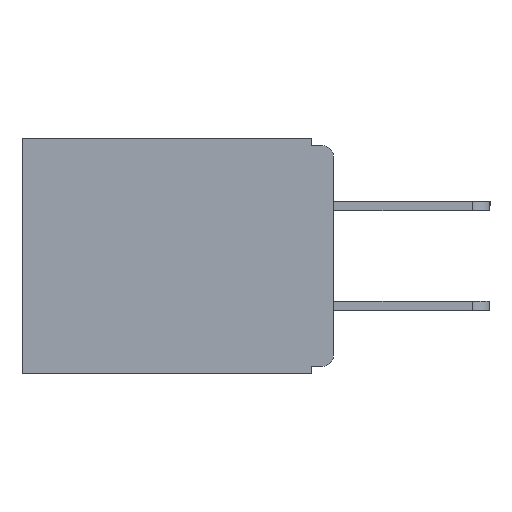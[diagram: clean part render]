
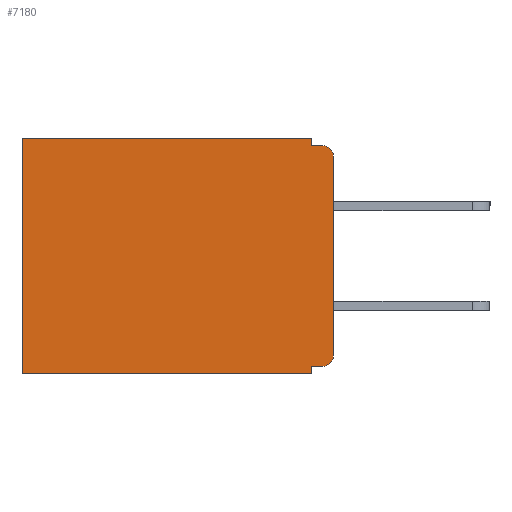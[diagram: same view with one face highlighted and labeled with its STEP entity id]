
A CAD part, left-side view. The second image highlights one B-rep face of the part: STEP entity #7180.
In plain terms, the highlighted planar face has unit normal (-1, 0, 0).
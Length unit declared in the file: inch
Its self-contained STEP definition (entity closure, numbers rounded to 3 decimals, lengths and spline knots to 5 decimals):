
#23 = ORIENTED_EDGE ( 'NONE', *, *, #28409, .T. ) ;
#309 = CARTESIAN_POINT ( 'NONE',  ( 0.3, 0.437, -0.33 ) ) ;
#776 = CARTESIAN_POINT ( 'NONE',  ( 0.3, 0., 0. ) ) ;
#1115 = EDGE_CURVE ( 'NONE', #1236, #22009, #10466, .T. ) ;
#1236 = VERTEX_POINT ( 'NONE', #13612 ) ;
#1358 = VECTOR ( 'NONE', #11368, 39.37008 ) ;
#1488 = EDGE_CURVE ( 'NONE', #31848, #22009, #25218, .T. ) ;
#2043 = VERTEX_POINT ( 'NONE', #20095 ) ;
#2338 = DIRECTION ( 'NONE',  ( 0., 0., -1. ) ) ;
#2841 = ORIENTED_EDGE ( 'NONE', *, *, #1115, .F. ) ;
#3226 = ORIENTED_EDGE ( 'NONE', *, *, #15788, .F. ) ;
#3723 = VERTEX_POINT ( 'NONE', #20321 ) ;
#4534 = PLANE ( 'NONE',  #27594 ) ;
#5352 = VECTOR ( 'NONE', #10375, 39.37008 ) ;
#5777 = EDGE_CURVE ( 'NONE', #2043, #10808, #27168, .T. ) ;
#6346 = ORIENTED_EDGE ( 'NONE', *, *, #23452, .T. ) ;
#6416 = CARTESIAN_POINT ( 'NONE',  ( 0.3, 0.015, -0.32 ) ) ;
#6568 = VECTOR ( 'NONE', #13003, 39.37008 ) ;
#6721 = VERTEX_POINT ( 'NONE', #17776 ) ;
#7156 = DIRECTION ( 'NONE',  ( 1., 0., 0. ) ) ;
#7180 = ADVANCED_FACE ( 'NONE', ( #17403 ), #4534, .F. ) ;
#7276 = CARTESIAN_POINT ( 'NONE',  ( 0.3, 0.031, 0. ) ) ;
#7958 = ORIENTED_EDGE ( 'NONE', *, *, #1488, .T. ) ;
#8324 = DIRECTION ( 'NONE',  ( -1., 0., 0. ) ) ;
#8443 = EDGE_CURVE ( 'NONE', #27253, #19172, #18539, .T. ) ;
#8876 = CARTESIAN_POINT ( 'NONE',  ( 0.3, 0.031, -0.33 ) ) ;
#9411 = CARTESIAN_POINT ( 'NONE',  ( 0.3, 0., -0.33 ) ) ;
#10375 = DIRECTION ( 'NONE',  ( 0., 0., -1. ) ) ;
#10466 = LINE ( 'NONE', #9411, #29503 ) ;
#10626 = VECTOR ( 'NONE', #27762, 39.37008 ) ;
#10808 = VERTEX_POINT ( 'NONE', #25411 ) ;
#10953 = CIRCLE ( 'NONE', #18537, 0.015 ) ;
#11368 = DIRECTION ( 'NONE',  ( 0., 0., -1. ) ) ;
#11423 = EDGE_LOOP ( 'NONE', ( #30454, #23, #3226, #14983, #6346, #7958, #2841, #24669, #26247, #23907 ) ) ;
#11524 = LINE ( 'NONE', #7276, #29790 ) ;
#12061 = CARTESIAN_POINT ( 'NONE',  ( 0.3, 0., -0.33 ) ) ;
#12395 = CARTESIAN_POINT ( 'NONE',  ( 0.3, 0.015, -0.305 ) ) ;
#12618 = AXIS2_PLACEMENT_3D ( 'NONE', #23200, #8324, #25711 ) ;
#12680 = CARTESIAN_POINT ( 'NONE',  ( 0.3, 0., -0.33 ) ) ;
#12694 = VECTOR ( 'NONE', #32144, 39.37008 ) ;
#13003 = DIRECTION ( 'NONE',  ( 0., 0., -1. ) ) ;
#13612 = CARTESIAN_POINT ( 'NONE',  ( 0.3, 0.031, -0.33 ) ) ;
#13890 = EDGE_CURVE ( 'NONE', #19172, #1236, #16249, .T. ) ;
#14872 = CARTESIAN_POINT ( 'NONE',  ( 0.3, 0., -0.32 ) ) ;
#14921 = DIRECTION ( 'NONE',  ( 0., 0., -1. ) ) ;
#14983 = ORIENTED_EDGE ( 'NONE', *, *, #23185, .F. ) ;
#15788 = EDGE_CURVE ( 'NONE', #6721, #27432, #23838, .T. ) ;
#16205 = VECTOR ( 'NONE', #28239, 39.37008 ) ;
#16249 = LINE ( 'NONE', #8876, #1358 ) ;
#17403 = FACE_OUTER_BOUND ( 'NONE', #11423, .T. ) ;
#17776 = CARTESIAN_POINT ( 'NONE',  ( 0.3, 0.031, -0.01 ) ) ;
#18537 = AXIS2_PLACEMENT_3D ( 'NONE', #12395, #29750, #14921 ) ;
#18539 = LINE ( 'NONE', #14872, #12694 ) ;
#19172 = VERTEX_POINT ( 'NONE', #29341 ) ;
#19593 = CARTESIAN_POINT ( 'NONE',  ( 0.3, 0.015, -0.01 ) ) ;
#20095 = CARTESIAN_POINT ( 'NONE',  ( 0.3, 0., -0.025 ) ) ;
#20321 = CARTESIAN_POINT ( 'NONE',  ( 0.3, 0.031, 0. ) ) ;
#20507 = CIRCLE ( 'NONE', #12618, 0.015 ) ;
#22009 = VERTEX_POINT ( 'NONE', #309 ) ;
#23185 = EDGE_CURVE ( 'NONE', #3723, #6721, #11524, .T. ) ;
#23200 = CARTESIAN_POINT ( 'NONE',  ( 0.3, 0.015, -0.025 ) ) ;
#23452 = EDGE_CURVE ( 'NONE', #3723, #31848, #23564, .T. ) ;
#23564 = LINE ( 'NONE', #776, #16205 ) ;
#23838 = LINE ( 'NONE', #25295, #10626 ) ;
#23907 = ORIENTED_EDGE ( 'NONE', *, *, #31975, .T. ) ;
#24545 = DIRECTION ( 'NONE',  ( 0., 0., -1. ) ) ;
#24669 = ORIENTED_EDGE ( 'NONE', *, *, #13890, .F. ) ;
#25218 = LINE ( 'NONE', #30579, #5352 ) ;
#25295 = CARTESIAN_POINT ( 'NONE',  ( 0.3, 0., -0.01 ) ) ;
#25411 = CARTESIAN_POINT ( 'NONE',  ( 0.3, 0., -0.305 ) ) ;
#25711 = DIRECTION ( 'NONE',  ( 0., 0., -1. ) ) ;
#26247 = ORIENTED_EDGE ( 'NONE', *, *, #8443, .F. ) ;
#27168 = LINE ( 'NONE', #12680, #6568 ) ;
#27253 = VERTEX_POINT ( 'NONE', #6416 ) ;
#27432 = VERTEX_POINT ( 'NONE', #19593 ) ;
#27594 = AXIS2_PLACEMENT_3D ( 'NONE', #12061, #7156, #24545 ) ;
#27762 = DIRECTION ( 'NONE',  ( 0., -1., 0. ) ) ;
#28239 = DIRECTION ( 'NONE',  ( 0., 1., 0. ) ) ;
#28409 = EDGE_CURVE ( 'NONE', #2043, #27432, #20507, .T. ) ;
#29101 = CARTESIAN_POINT ( 'NONE',  ( 0.3, 0.437, 0. ) ) ;
#29341 = CARTESIAN_POINT ( 'NONE',  ( 0.3, 0.031, -0.32 ) ) ;
#29503 = VECTOR ( 'NONE', #30112, 39.37008 ) ;
#29750 = DIRECTION ( 'NONE',  ( -1., 0., 0. ) ) ;
#29790 = VECTOR ( 'NONE', #2338, 39.37008 ) ;
#30112 = DIRECTION ( 'NONE',  ( 0., 1., 0. ) ) ;
#30454 = ORIENTED_EDGE ( 'NONE', *, *, #5777, .F. ) ;
#30579 = CARTESIAN_POINT ( 'NONE',  ( 0.3, 0.437, -0.33 ) ) ;
#31848 = VERTEX_POINT ( 'NONE', #29101 ) ;
#31975 = EDGE_CURVE ( 'NONE', #27253, #10808, #10953, .T. ) ;
#32144 = DIRECTION ( 'NONE',  ( 0., 1., 0. ) ) ;
